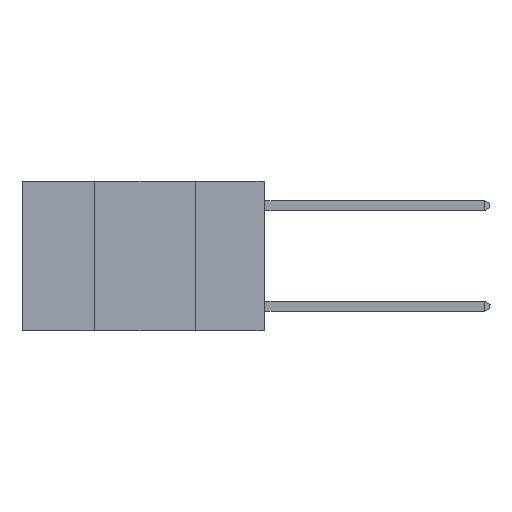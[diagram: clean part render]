
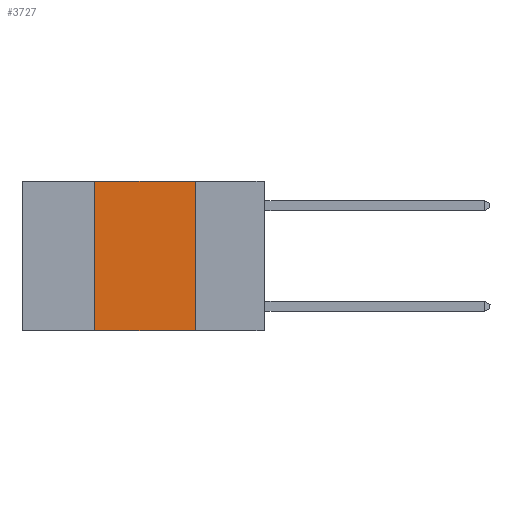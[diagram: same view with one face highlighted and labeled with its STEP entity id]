
A CAD part, left-side view. The second image highlights one B-rep face of the part: STEP entity #3727.
In plain terms, the highlighted planar face has unit normal (-1, 0, 0).
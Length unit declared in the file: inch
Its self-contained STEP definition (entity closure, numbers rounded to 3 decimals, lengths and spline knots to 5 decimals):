
#679 = DIRECTION ( 'NONE',  ( 0., 0., -1. ) ) ;
#2019 = DIRECTION ( 'NONE',  ( 0., -1., 0. ) ) ;
#2047 = VERTEX_POINT ( 'NONE', #13403 ) ;
#2302 = CARTESIAN_POINT ( 'NONE',  ( 0., 0.6, 0. ) ) ;
#2384 = CARTESIAN_POINT ( 'NONE',  ( 0., 0.42, 0. ) ) ;
#3159 = VECTOR ( 'NONE', #18956, 39.37008 ) ;
#3727 = ADVANCED_FACE ( 'NONE', ( #15259 ), #11305, .F. ) ;
#3853 = DIRECTION ( 'NONE',  ( 0., 0., -1. ) ) ;
#4929 = CARTESIAN_POINT ( 'NONE',  ( 0., 0.17, 0. ) ) ;
#5366 = EDGE_LOOP ( 'NONE', ( #19050, #17131, #15081, #17591 ) ) ;
#6663 = CARTESIAN_POINT ( 'NONE',  ( 0., 0.17, 0. ) ) ;
#7156 = LINE ( 'NONE', #2384, #3159 ) ;
#7410 = EDGE_CURVE ( 'NONE', #8641, #11405, #17677, .T. ) ;
#8058 = CARTESIAN_POINT ( 'NONE',  ( 0., 0.6, -0.37 ) ) ;
#8641 = VERTEX_POINT ( 'NONE', #4929 ) ;
#10566 = VECTOR ( 'NONE', #16456, 39.37008 ) ;
#11023 = LINE ( 'NONE', #11952, #10566 ) ;
#11092 = VECTOR ( 'NONE', #2019, 39.37008 ) ;
#11305 = PLANE ( 'NONE',  #19148 ) ;
#11405 = VERTEX_POINT ( 'NONE', #18768 ) ;
#11952 = CARTESIAN_POINT ( 'NONE',  ( 0., 0.6, 0. ) ) ;
#12827 = DIRECTION ( 'NONE',  ( 1., 0., 0. ) ) ;
#13403 = CARTESIAN_POINT ( 'NONE',  ( 0., 0.42, 0. ) ) ;
#14176 = EDGE_CURVE ( 'NONE', #18069, #2047, #7156, .T. ) ;
#15081 = ORIENTED_EDGE ( 'NONE', *, *, #14176, .F. ) ;
#15259 = FACE_OUTER_BOUND ( 'NONE', #5366, .T. ) ;
#15874 = EDGE_CURVE ( 'NONE', #18069, #11405, #19081, .T. ) ;
#16456 = DIRECTION ( 'NONE',  ( 0., -1., 0. ) ) ;
#16949 = EDGE_CURVE ( 'NONE', #2047, #8641, #11023, .T. ) ;
#17131 = ORIENTED_EDGE ( 'NONE', *, *, #16949, .F. ) ;
#17196 = VECTOR ( 'NONE', #679, 39.37008 ) ;
#17591 = ORIENTED_EDGE ( 'NONE', *, *, #15874, .T. ) ;
#17677 = LINE ( 'NONE', #6663, #17196 ) ;
#17687 = CARTESIAN_POINT ( 'NONE',  ( 0., 0.42, -0.37 ) ) ;
#18069 = VERTEX_POINT ( 'NONE', #17687 ) ;
#18768 = CARTESIAN_POINT ( 'NONE',  ( 0., 0.17, -0.37 ) ) ;
#18956 = DIRECTION ( 'NONE',  ( 0., 0., 1. ) ) ;
#19050 = ORIENTED_EDGE ( 'NONE', *, *, #7410, .F. ) ;
#19081 = LINE ( 'NONE', #8058, #11092 ) ;
#19148 = AXIS2_PLACEMENT_3D ( 'NONE', #2302, #12827, #3853 ) ;
